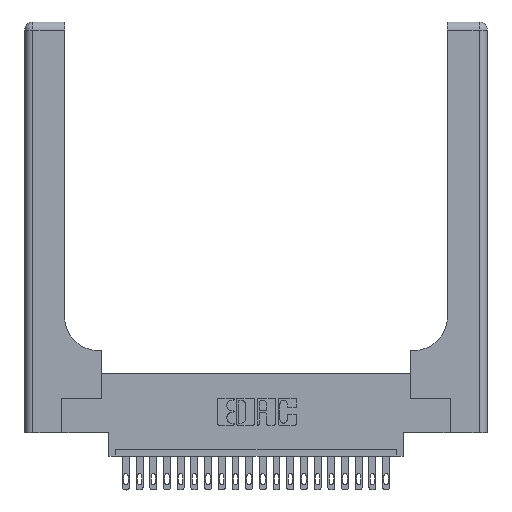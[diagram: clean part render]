
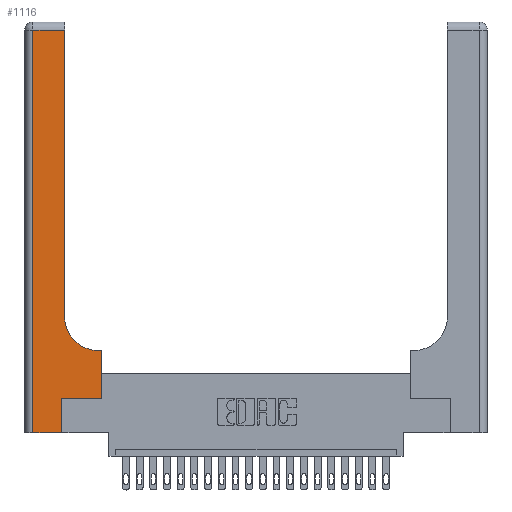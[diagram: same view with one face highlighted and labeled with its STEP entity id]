
A CAD part, top view. The second image highlights one B-rep face of the part: STEP entity #1116.
In plain terms, the highlighted planar face has unit normal (0, 0, 1).
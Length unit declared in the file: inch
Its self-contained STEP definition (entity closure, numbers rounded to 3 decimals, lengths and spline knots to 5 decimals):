
#329 = DIRECTION ( 'NONE',  ( 0., 1., 0. ) ) ;
#1116 = ADVANCED_FACE ( 'NONE', ( #12455 ), #5536, .F. ) ;
#1287 = EDGE_LOOP ( 'NONE', ( #9076, #8962, #4789, #21440, #20473, #12132, #23179, #5028, #21768 ) ) ;
#1477 = CARTESIAN_POINT ( 'NONE',  ( 0.2915, 0.85, 0.37 ) ) ;
#1601 = LINE ( 'NONE', #18763, #22082 ) ;
#2552 = CARTESIAN_POINT ( 'NONE',  ( 0.06, 2.94, 0.37 ) ) ;
#3245 = CARTESIAN_POINT ( 'NONE',  ( 0.5415, 0.85, 0.37 ) ) ;
#3267 = LINE ( 'NONE', #17398, #9778 ) ;
#3358 = CARTESIAN_POINT ( 'NONE',  ( 0.5415, 0.6, 0.37 ) ) ;
#4158 = EDGE_CURVE ( 'NONE', #13682, #17350, #3267, .T. ) ;
#4346 = CARTESIAN_POINT ( 'NONE',  ( 0.2915, 0.6, 0.37 ) ) ;
#4569 = CARTESIAN_POINT ( 'NONE',  ( 0.2915, 3., 0.37 ) ) ;
#4789 = ORIENTED_EDGE ( 'NONE', *, *, #14256, .T. ) ;
#4829 = VECTOR ( 'NONE', #22852, 39.37008 ) ;
#5028 = ORIENTED_EDGE ( 'NONE', *, *, #10465, .T. ) ;
#5170 = VERTEX_POINT ( 'NONE', #6868 ) ;
#5247 = VECTOR ( 'NONE', #7987, 39.37008 ) ;
#5536 = PLANE ( 'NONE',  #18448 ) ;
#5812 = VERTEX_POINT ( 'NONE', #14883 ) ;
#6036 = DIRECTION ( 'NONE',  ( 0., -1., 0. ) ) ;
#6167 = CARTESIAN_POINT ( 'NONE',  ( 0.06, 0., 0.37 ) ) ;
#6292 = AXIS2_PLACEMENT_3D ( 'NONE', #3245, #6790, #8616 ) ;
#6487 = CARTESIAN_POINT ( 'NONE',  ( 0.269, 0.25, 0.37 ) ) ;
#6790 = DIRECTION ( 'NONE',  ( 0., 0., -1. ) ) ;
#6868 = CARTESIAN_POINT ( 'NONE',  ( 0.5585, 0.6, 0.37 ) ) ;
#7867 = VERTEX_POINT ( 'NONE', #3358 ) ;
#7943 = CARTESIAN_POINT ( 'NONE',  ( 0., 0., 0.37 ) ) ;
#7987 = DIRECTION ( 'NONE',  ( -1., 0., 0. ) ) ;
#8380 = VERTEX_POINT ( 'NONE', #6167 ) ;
#8616 = DIRECTION ( 'NONE',  ( 1., 0., 0. ) ) ;
#8847 = VECTOR ( 'NONE', #16830, 39.37008 ) ;
#8962 = ORIENTED_EDGE ( 'NONE', *, *, #4158, .T. ) ;
#8987 = VECTOR ( 'NONE', #11712, 39.37008 ) ;
#9076 = ORIENTED_EDGE ( 'NONE', *, *, #21570, .T. ) ;
#9301 = EDGE_CURVE ( 'NONE', #7867, #22327, #12040, .T. ) ;
#9662 = LINE ( 'NONE', #16329, #14427 ) ;
#9691 = EDGE_CURVE ( 'NONE', #8380, #11749, #17671, .T. ) ;
#9778 = VECTOR ( 'NONE', #17346, 39.37008 ) ;
#9830 = CARTESIAN_POINT ( 'NONE',  ( 0.269, 0.25, 0.37 ) ) ;
#10272 = EDGE_CURVE ( 'NONE', #5812, #5170, #1601, .T. ) ;
#10465 = EDGE_CURVE ( 'NONE', #5170, #7867, #10629, .T. ) ;
#10629 = LINE ( 'NONE', #4346, #5247 ) ;
#10756 = DIRECTION ( 'NONE',  ( 0., 0., -1. ) ) ;
#11401 = CARTESIAN_POINT ( 'NONE',  ( 0.06, 3., 0.37 ) ) ;
#11625 = LINE ( 'NONE', #4569, #4829 ) ;
#11712 = DIRECTION ( 'NONE',  ( 1., 0., 0. ) ) ;
#11749 = VERTEX_POINT ( 'NONE', #12477 ) ;
#12040 = CIRCLE ( 'NONE', #6292, 0.25 ) ;
#12132 = ORIENTED_EDGE ( 'NONE', *, *, #14223, .T. ) ;
#12455 = FACE_OUTER_BOUND ( 'NONE', #1287, .T. ) ;
#12477 = CARTESIAN_POINT ( 'NONE',  ( 0.269, 0., 0.37 ) ) ;
#12806 = VECTOR ( 'NONE', #6036, 39.37008 ) ;
#13627 = VERTEX_POINT ( 'NONE', #6487 ) ;
#13682 = VERTEX_POINT ( 'NONE', #14117 ) ;
#14117 = CARTESIAN_POINT ( 'NONE',  ( 0.2915, 2.94, 0.37 ) ) ;
#14223 = EDGE_CURVE ( 'NONE', #13627, #5812, #15872, .T. ) ;
#14256 = EDGE_CURVE ( 'NONE', #17350, #8380, #17566, .T. ) ;
#14427 = VECTOR ( 'NONE', #329, 39.37008 ) ;
#14883 = CARTESIAN_POINT ( 'NONE',  ( 0.5585, 0.25, 0.37 ) ) ;
#15346 = EDGE_CURVE ( 'NONE', #11749, #13627, #9662, .T. ) ;
#15872 = LINE ( 'NONE', #9830, #8847 ) ;
#16329 = CARTESIAN_POINT ( 'NONE',  ( 0.269, 0., 0.37 ) ) ;
#16830 = DIRECTION ( 'NONE',  ( 1., 0., 0. ) ) ;
#17346 = DIRECTION ( 'NONE',  ( -1., 0., 0. ) ) ;
#17350 = VERTEX_POINT ( 'NONE', #2552 ) ;
#17398 = CARTESIAN_POINT ( 'NONE',  ( 0., 2.94, 0.37 ) ) ;
#17566 = LINE ( 'NONE', #11401, #12806 ) ;
#17671 = LINE ( 'NONE', #7943, #8987 ) ;
#18120 = DIRECTION ( 'NONE',  ( -1., 0., 0. ) ) ;
#18448 = AXIS2_PLACEMENT_3D ( 'NONE', #21689, #10756, #18120 ) ;
#18763 = CARTESIAN_POINT ( 'NONE',  ( 0.5585, 0.25, 0.37 ) ) ;
#20473 = ORIENTED_EDGE ( 'NONE', *, *, #15346, .T. ) ;
#21440 = ORIENTED_EDGE ( 'NONE', *, *, #9691, .T. ) ;
#21570 = EDGE_CURVE ( 'NONE', #22327, #13682, #11625, .T. ) ;
#21689 = CARTESIAN_POINT ( 'NONE',  ( 0., 3., 0.37 ) ) ;
#21768 = ORIENTED_EDGE ( 'NONE', *, *, #9301, .T. ) ;
#22082 = VECTOR ( 'NONE', #22551, 39.37008 ) ;
#22327 = VERTEX_POINT ( 'NONE', #1477 ) ;
#22551 = DIRECTION ( 'NONE',  ( 0., 1., 0. ) ) ;
#22852 = DIRECTION ( 'NONE',  ( 0., 1., 0. ) ) ;
#23179 = ORIENTED_EDGE ( 'NONE', *, *, #10272, .T. ) ;
